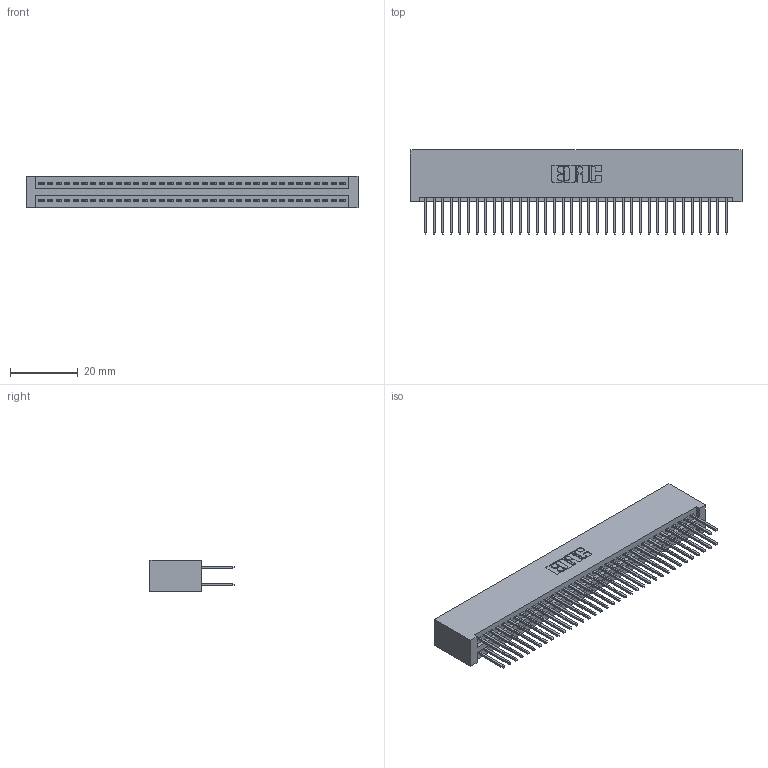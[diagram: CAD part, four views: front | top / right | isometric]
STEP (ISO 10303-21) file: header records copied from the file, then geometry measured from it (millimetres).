
FILE_DESCRIPTION (( 'STEP AP203' ), '1' );
FILE_NAME ('345-072-523-201.STEP', '2018-10-02T04:23:09', ( '' ), ( '' ), 'SwSTEP 2.0', 'SolidWorks 2016', '' );
FILE_SCHEMA (( 'CONFIG_CONTROL_DESIGN' ));
Length unit declared in the file: inch
Products named in the file (3): 345-072-523-201; 345 Part_No Mounting Lugs; 345-292-001_345-293-123
Assembly tree (73 placements, depth 2):
  345-072-523-201
    345 Part_No Mounting Lugs
    345-292-001_345-293-123  x72
Bounding box: 98.04 x 24.82 x 9.4 mm (x, y, z)
Volume: 10231.9 mm3; surface area: 15973.5 mm2
Topology: 73 solids, 73 shells, 3718 faces, 11045 edges, 7266 vertices
Faces by surface type: plane 2452, cylinder 1266
Entity records: 28795 total; most frequent: CARTESIAN_POINT 4832, ORIENTED_EDGE 4766, DIRECTION 4263, EDGE_CURVE 2383, LINE 2115, VECTOR 2115, VERTEX_POINT 1586, AXIS2_PLACEMENT_3D 1074
